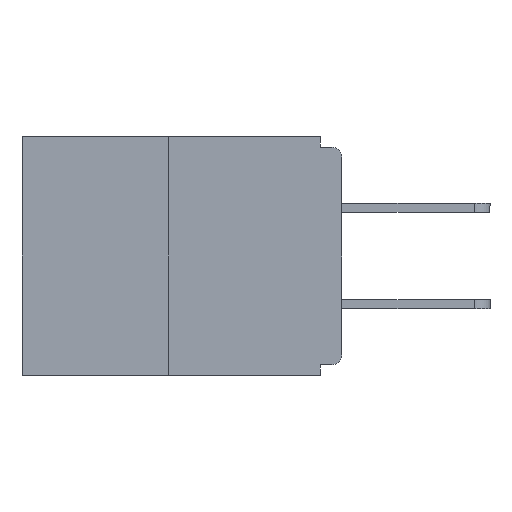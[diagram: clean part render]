
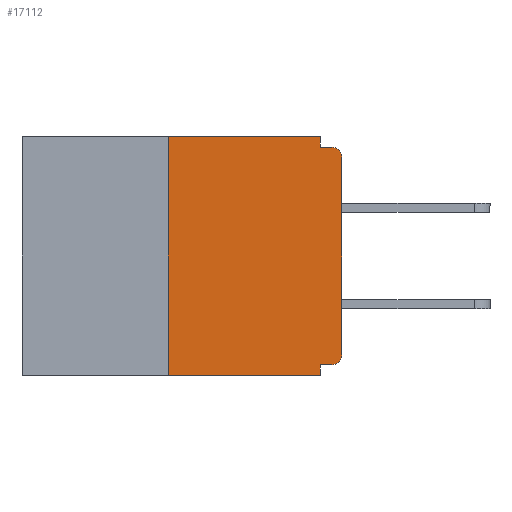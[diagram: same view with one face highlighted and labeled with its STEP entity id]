
A CAD part, left-side view. The second image highlights one B-rep face of the part: STEP entity #17112.
In plain terms, the highlighted planar face has unit normal (-1, 0, 0).
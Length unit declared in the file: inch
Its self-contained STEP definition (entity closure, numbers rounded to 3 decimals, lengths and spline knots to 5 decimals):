
#107 = AXIS2_PLACEMENT_3D ( 'NONE', #905, #11575, #17176 ) ;
#364 = VECTOR ( 'NONE', #5668, 39.37008 ) ;
#793 = CIRCLE ( 'NONE', #10844, 0.015 ) ;
#905 = CARTESIAN_POINT ( 'NONE',  ( 0., 0.015, -0.313 ) ) ;
#1019 = CARTESIAN_POINT ( 'NONE',  ( 0., 0., -0.328 ) ) ;
#1021 = VECTOR ( 'NONE', #11082, 39.37008 ) ;
#1272 = CARTESIAN_POINT ( 'NONE',  ( 0., 0.25, 0. ) ) ;
#1683 = CARTESIAN_POINT ( 'NONE',  ( 0., 0.015, -0.328 ) ) ;
#1800 = VECTOR ( 'NONE', #17265, 39.37008 ) ;
#2484 = EDGE_CURVE ( 'NONE', #4187, #11749, #9932, .T. ) ;
#2580 = VECTOR ( 'NONE', #6398, 39.37008 ) ;
#2716 = DIRECTION ( 'NONE',  ( 0., 1., 0. ) ) ;
#2979 = VERTEX_POINT ( 'NONE', #18177 ) ;
#3386 = PLANE ( 'NONE',  #5720 ) ;
#3599 = VERTEX_POINT ( 'NONE', #15250 ) ;
#3661 = EDGE_CURVE ( 'NONE', #4974, #2979, #13910, .T. ) ;
#3899 = VECTOR ( 'NONE', #8910, 39.37008 ) ;
#3909 = DIRECTION ( 'NONE',  ( 0., -1., 0. ) ) ;
#4187 = VERTEX_POINT ( 'NONE', #13791 ) ;
#4489 = EDGE_CURVE ( 'NONE', #14743, #17765, #12997, .T. ) ;
#4831 = LINE ( 'NONE', #1272, #11252 ) ;
#4962 = CIRCLE ( 'NONE', #107, 0.015 ) ;
#4974 = VERTEX_POINT ( 'NONE', #1683 ) ;
#5226 = ORIENTED_EDGE ( 'NONE', *, *, #3661, .F. ) ;
#5668 = DIRECTION ( 'NONE',  ( 0., 0., -1. ) ) ;
#5720 = AXIS2_PLACEMENT_3D ( 'NONE', #17686, #7595, #9036 ) ;
#6398 = DIRECTION ( 'NONE',  ( 0., 0., 1. ) ) ;
#7537 = ORIENTED_EDGE ( 'NONE', *, *, #11479, .T. ) ;
#7595 = DIRECTION ( 'NONE',  ( 1., 0., 0. ) ) ;
#7966 = LINE ( 'NONE', #15317, #364 ) ;
#8217 = CARTESIAN_POINT ( 'NONE',  ( 0., 0.25, 0. ) ) ;
#8297 = EDGE_CURVE ( 'NONE', #4974, #4187, #4962, .T. ) ;
#8641 = VERTEX_POINT ( 'NONE', #9985 ) ;
#8910 = DIRECTION ( 'NONE',  ( 0., -1., 0. ) ) ;
#8956 = ORIENTED_EDGE ( 'NONE', *, *, #16748, .F. ) ;
#8972 = VECTOR ( 'NONE', #3909, 39.37008 ) ;
#9036 = DIRECTION ( 'NONE',  ( 0., 0., -1. ) ) ;
#9273 = CARTESIAN_POINT ( 'NONE',  ( 0., 0., 0. ) ) ;
#9462 = VERTEX_POINT ( 'NONE', #14338 ) ;
#9511 = LINE ( 'NONE', #15187, #1021 ) ;
#9819 = LINE ( 'NONE', #12164, #8972 ) ;
#9932 = LINE ( 'NONE', #9273, #2580 ) ;
#9985 = CARTESIAN_POINT ( 'NONE',  ( 0., 0.031, -0.015 ) ) ;
#10262 = CARTESIAN_POINT ( 'NONE',  ( 0., 0.46, 0. ) ) ;
#10473 = ORIENTED_EDGE ( 'NONE', *, *, #13803, .F. ) ;
#10784 = ORIENTED_EDGE ( 'NONE', *, *, #11127, .F. ) ;
#10844 = AXIS2_PLACEMENT_3D ( 'NONE', #15897, #13043, #17335 ) ;
#11082 = DIRECTION ( 'NONE',  ( 0., -1., 0. ) ) ;
#11127 = EDGE_CURVE ( 'NONE', #8641, #14544, #9511, .T. ) ;
#11183 = CARTESIAN_POINT ( 'NONE',  ( 0., 0., -0.03 ) ) ;
#11252 = VECTOR ( 'NONE', #15533, 39.37008 ) ;
#11378 = EDGE_CURVE ( 'NONE', #3599, #14743, #4831, .T. ) ;
#11462 = CARTESIAN_POINT ( 'NONE',  ( 0., 0.031, -0.343 ) ) ;
#11479 = EDGE_CURVE ( 'NONE', #11749, #14544, #793, .T. ) ;
#11575 = DIRECTION ( 'NONE',  ( -1., 0., 0. ) ) ;
#11749 = VERTEX_POINT ( 'NONE', #11183 ) ;
#12028 = FACE_OUTER_BOUND ( 'NONE', #14929, .T. ) ;
#12070 = CARTESIAN_POINT ( 'NONE',  ( 0., 0.031, 0. ) ) ;
#12164 = CARTESIAN_POINT ( 'NONE',  ( 0., 0.46, -0.343 ) ) ;
#12997 = LINE ( 'NONE', #10262, #3899 ) ;
#13043 = DIRECTION ( 'NONE',  ( -1., 0., 0. ) ) ;
#13791 = CARTESIAN_POINT ( 'NONE',  ( 0., 0., -0.313 ) ) ;
#13803 = EDGE_CURVE ( 'NONE', #17765, #8641, #7966, .T. ) ;
#13910 = LINE ( 'NONE', #1019, #18381 ) ;
#14338 = CARTESIAN_POINT ( 'NONE',  ( 0., 0.031, -0.343 ) ) ;
#14544 = VERTEX_POINT ( 'NONE', #17553 ) ;
#14743 = VERTEX_POINT ( 'NONE', #8217 ) ;
#14890 = ORIENTED_EDGE ( 'NONE', *, *, #4489, .F. ) ;
#14929 = EDGE_LOOP ( 'NONE', ( #14890, #16971, #16875, #8956, #5226, #17128, #16642, #7537, #10784, #10473 ) ) ;
#15187 = CARTESIAN_POINT ( 'NONE',  ( 0., 0., -0.015 ) ) ;
#15250 = CARTESIAN_POINT ( 'NONE',  ( 0., 0.25, -0.343 ) ) ;
#15317 = CARTESIAN_POINT ( 'NONE',  ( 0., 0.031, 0. ) ) ;
#15533 = DIRECTION ( 'NONE',  ( 0., 0., 1. ) ) ;
#15897 = CARTESIAN_POINT ( 'NONE',  ( 0., 0.015, -0.03 ) ) ;
#16481 = EDGE_CURVE ( 'NONE', #3599, #9462, #9819, .T. ) ;
#16642 = ORIENTED_EDGE ( 'NONE', *, *, #2484, .T. ) ;
#16709 = LINE ( 'NONE', #11462, #1800 ) ;
#16748 = EDGE_CURVE ( 'NONE', #2979, #9462, #16709, .T. ) ;
#16875 = ORIENTED_EDGE ( 'NONE', *, *, #16481, .T. ) ;
#16971 = ORIENTED_EDGE ( 'NONE', *, *, #11378, .F. ) ;
#17112 = ADVANCED_FACE ( 'NONE', ( #12028 ), #3386, .F. ) ;
#17128 = ORIENTED_EDGE ( 'NONE', *, *, #8297, .T. ) ;
#17176 = DIRECTION ( 'NONE',  ( 0., 0., -1. ) ) ;
#17265 = DIRECTION ( 'NONE',  ( 0., 0., -1. ) ) ;
#17335 = DIRECTION ( 'NONE',  ( 0., 0., -1. ) ) ;
#17553 = CARTESIAN_POINT ( 'NONE',  ( 0., 0.015, -0.015 ) ) ;
#17686 = CARTESIAN_POINT ( 'NONE',  ( 0., 0.46, 0. ) ) ;
#17765 = VERTEX_POINT ( 'NONE', #12070 ) ;
#18177 = CARTESIAN_POINT ( 'NONE',  ( 0., 0.031, -0.328 ) ) ;
#18381 = VECTOR ( 'NONE', #2716, 39.37008 ) ;
